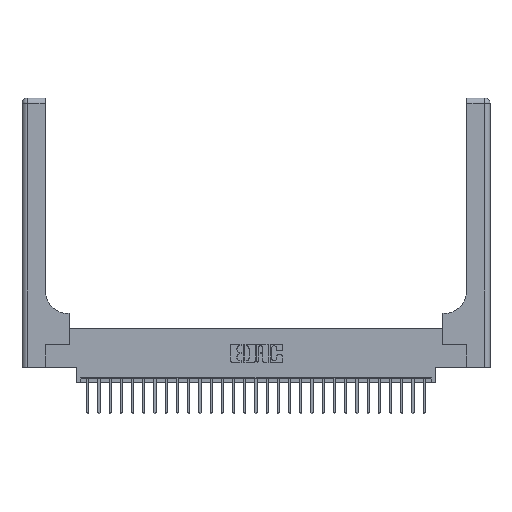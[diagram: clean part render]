
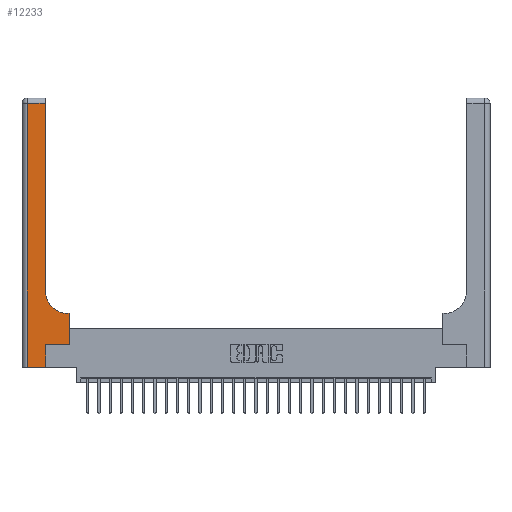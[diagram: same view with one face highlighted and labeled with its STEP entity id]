
A CAD part, top view. The second image highlights one B-rep face of the part: STEP entity #12233.
In plain terms, the highlighted planar face has unit normal (0, 0, 1).
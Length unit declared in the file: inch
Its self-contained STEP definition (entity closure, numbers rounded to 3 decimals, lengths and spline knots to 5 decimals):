
#220 = CARTESIAN_POINT ( 'NONE',  ( 0.06, 3., 0.37 ) ) ;
#330 = AXIS2_PLACEMENT_3D ( 'NONE', #2864, #17532, #5018 ) ;
#398 = VECTOR ( 'NONE', #717, 39.37008 ) ;
#509 = DIRECTION ( 'NONE',  ( 1., 0., 0. ) ) ;
#622 = ORIENTED_EDGE ( 'NONE', *, *, #21236, .T. ) ;
#717 = DIRECTION ( 'NONE',  ( -1., 0., 0. ) ) ;
#783 = PLANE ( 'NONE',  #330 ) ;
#1070 = LINE ( 'NONE', #13282, #398 ) ;
#1124 = LINE ( 'NONE', #220, #22726 ) ;
#1285 = LINE ( 'NONE', #20024, #11802 ) ;
#1501 = EDGE_CURVE ( 'NONE', #11807, #12183, #13795, .T. ) ;
#1951 = VERTEX_POINT ( 'NONE', #15348 ) ;
#2023 = EDGE_CURVE ( 'NONE', #14347, #6217, #1285, .T. ) ;
#2546 = EDGE_CURVE ( 'NONE', #24799, #14347, #6865, .T. ) ;
#2864 = CARTESIAN_POINT ( 'NONE',  ( 0., 3., 0.37 ) ) ;
#3163 = AXIS2_PLACEMENT_3D ( 'NONE', #9013, #23620, #11129 ) ;
#3231 = DIRECTION ( 'NONE',  ( 0., 1., 0. ) ) ;
#3529 = CARTESIAN_POINT ( 'NONE',  ( 0.528, 0.25, 0.37 ) ) ;
#3617 = ORIENTED_EDGE ( 'NONE', *, *, #1501, .T. ) ;
#3771 = EDGE_LOOP ( 'NONE', ( #5772, #6193, #11297, #10379, #25615, #14275, #3617, #622, #19371 ) ) ;
#3772 = CARTESIAN_POINT ( 'NONE',  ( 0.51, 0.6, 0.37 ) ) ;
#4084 = CARTESIAN_POINT ( 'NONE',  ( 0.26, 2.94, 0.37 ) ) ;
#4699 = CARTESIAN_POINT ( 'NONE',  ( 0., 2.94, 0.37 ) ) ;
#5018 = DIRECTION ( 'NONE',  ( -1., 0., 0. ) ) ;
#5175 = CARTESIAN_POINT ( 'NONE',  ( 0.265, 0., 0.37 ) ) ;
#5395 = DIRECTION ( 'NONE',  ( 0., 1., 0. ) ) ;
#5772 = ORIENTED_EDGE ( 'NONE', *, *, #2023, .T. ) ;
#6193 = ORIENTED_EDGE ( 'NONE', *, *, #11024, .T. ) ;
#6217 = VERTEX_POINT ( 'NONE', #4084 ) ;
#6865 = CIRCLE ( 'NONE', #3163, 0.25 ) ;
#7563 = VECTOR ( 'NONE', #16080, 39.37008 ) ;
#8044 = CARTESIAN_POINT ( 'NONE',  ( 0.26, 0.85, 0.37 ) ) ;
#8864 = CARTESIAN_POINT ( 'NONE',  ( 0., 0., 0.37 ) ) ;
#8919 = DIRECTION ( 'NONE',  ( -1., 0., 0. ) ) ;
#9013 = CARTESIAN_POINT ( 'NONE',  ( 0.51, 0.85, 0.37 ) ) ;
#9335 = LINE ( 'NONE', #8864, #12941 ) ;
#9856 = VERTEX_POINT ( 'NONE', #15282 ) ;
#9943 = EDGE_CURVE ( 'NONE', #25286, #9856, #19104, .T. ) ;
#10379 = ORIENTED_EDGE ( 'NONE', *, *, #19808, .T. ) ;
#10775 = DIRECTION ( 'NONE',  ( 0., -1., 0. ) ) ;
#11024 = EDGE_CURVE ( 'NONE', #6217, #1951, #21998, .T. ) ;
#11129 = DIRECTION ( 'NONE',  ( 1., 0., 0. ) ) ;
#11297 = ORIENTED_EDGE ( 'NONE', *, *, #26882, .T. ) ;
#11802 = VECTOR ( 'NONE', #3231, 39.37008 ) ;
#11807 = VERTEX_POINT ( 'NONE', #24475 ) ;
#12183 = VERTEX_POINT ( 'NONE', #17264 ) ;
#12233 = ADVANCED_FACE ( 'NONE', ( #26805 ), #783, .F. ) ;
#12920 = CARTESIAN_POINT ( 'NONE',  ( 0.265, 0.25, 0.37 ) ) ;
#12941 = VECTOR ( 'NONE', #509, 39.37008 ) ;
#13282 = CARTESIAN_POINT ( 'NONE',  ( 0.26, 0.6, 0.37 ) ) ;
#13795 = LINE ( 'NONE', #3529, #7563 ) ;
#14275 = ORIENTED_EDGE ( 'NONE', *, *, #24353, .T. ) ;
#14347 = VERTEX_POINT ( 'NONE', #8044 ) ;
#15282 = CARTESIAN_POINT ( 'NONE',  ( 0.265, 0.25, 0.37 ) ) ;
#15348 = CARTESIAN_POINT ( 'NONE',  ( 0.06, 2.94, 0.37 ) ) ;
#15822 = CARTESIAN_POINT ( 'NONE',  ( 0.265, 0., 0.37 ) ) ;
#16080 = DIRECTION ( 'NONE',  ( 0., 1., 0. ) ) ;
#16402 = VECTOR ( 'NONE', #8919, 39.37008 ) ;
#16768 = VERTEX_POINT ( 'NONE', #21239 ) ;
#16983 = VECTOR ( 'NONE', #21229, 39.37008 ) ;
#17264 = CARTESIAN_POINT ( 'NONE',  ( 0.528, 0.6, 0.37 ) ) ;
#17532 = DIRECTION ( 'NONE',  ( 0., 0., -1. ) ) ;
#18433 = VECTOR ( 'NONE', #5395, 39.37008 ) ;
#19104 = LINE ( 'NONE', #15822, #18433 ) ;
#19371 = ORIENTED_EDGE ( 'NONE', *, *, #2546, .T. ) ;
#19808 = EDGE_CURVE ( 'NONE', #16768, #25286, #9335, .T. ) ;
#20024 = CARTESIAN_POINT ( 'NONE',  ( 0.26, 3., 0.37 ) ) ;
#21229 = DIRECTION ( 'NONE',  ( 1., 0., 0. ) ) ;
#21236 = EDGE_CURVE ( 'NONE', #12183, #24799, #1070, .T. ) ;
#21239 = CARTESIAN_POINT ( 'NONE',  ( 0.06, 0., 0.37 ) ) ;
#21916 = LINE ( 'NONE', #12920, #16983 ) ;
#21998 = LINE ( 'NONE', #4699, #16402 ) ;
#22726 = VECTOR ( 'NONE', #10775, 39.37008 ) ;
#23620 = DIRECTION ( 'NONE',  ( 0., 0., -1. ) ) ;
#24353 = EDGE_CURVE ( 'NONE', #9856, #11807, #21916, .T. ) ;
#24475 = CARTESIAN_POINT ( 'NONE',  ( 0.528, 0.25, 0.37 ) ) ;
#24799 = VERTEX_POINT ( 'NONE', #3772 ) ;
#25286 = VERTEX_POINT ( 'NONE', #5175 ) ;
#25615 = ORIENTED_EDGE ( 'NONE', *, *, #9943, .T. ) ;
#26805 = FACE_OUTER_BOUND ( 'NONE', #3771, .T. ) ;
#26882 = EDGE_CURVE ( 'NONE', #1951, #16768, #1124, .T. ) ;
